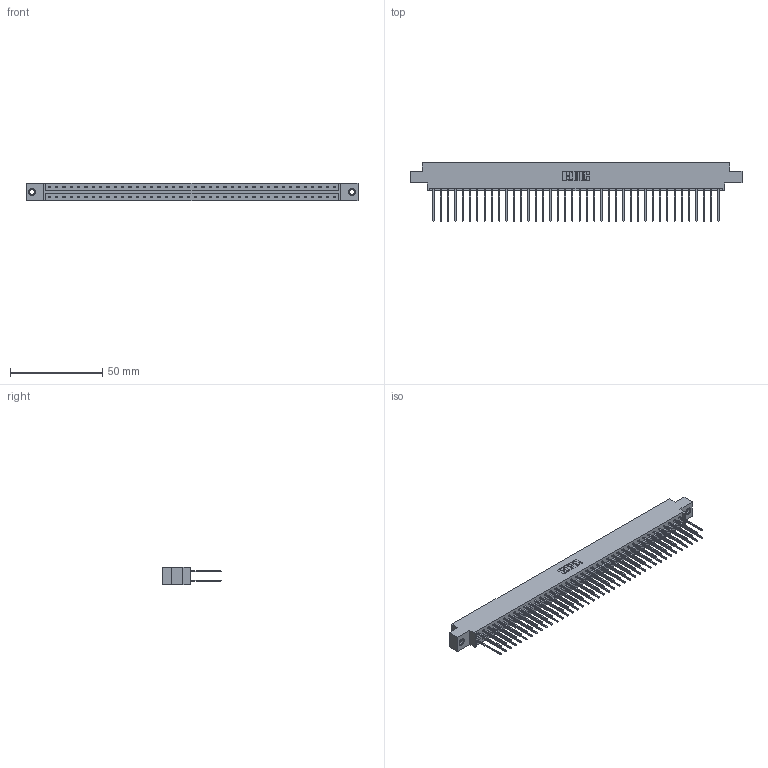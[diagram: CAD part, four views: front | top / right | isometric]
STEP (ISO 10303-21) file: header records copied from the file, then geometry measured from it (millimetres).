
FILE_DESCRIPTION (( 'STEP AP203' ), '1' );
FILE_NAME ('833-080-542-807.STEP', '2020-06-05T22:03:37', ( '' ), ( '' ), 'SwSTEP 2.0', 'SolidWorks 2020', '' );
FILE_SCHEMA (( 'CONFIG_CONTROL_DESIGN' ));
Length unit declared in the file: inch
Products named in the file (4): 345-292-001_345-293-142; 833 Part_Offset - .156 Dia - TI; 833-080-542-807; 345-250-001_345-250-005-103
Assembly tree (83 placements, depth 2):
  833-080-542-807
    833 Part_Offset - .156 Dia - TI
    345-292-001_345-293-142  x80
    345-250-001_345-250-005-103  x2
Bounding box: 180.04 x 31.63 x 9.4 mm (x, y, z)
Volume: 18493.5 mm3; surface area: 23942.6 mm2
Topology: 83 solids, 83 shells, 4338 faces, 12859 edges, 8458 vertices
Faces by surface type: plane 2986, cylinder 1336, cone 12, torus 4
Entity records: 27328 total; most frequent: CARTESIAN_POINT 4517, ORIENTED_EDGE 4446, DIRECTION 3893, EDGE_CURVE 2223, VECTOR 2075, LINE 2075, VERTEX_POINT 1476, AXIS2_PLACEMENT_3D 909
